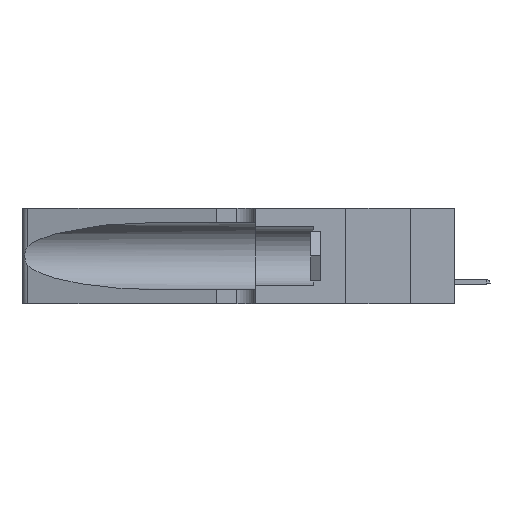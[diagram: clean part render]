
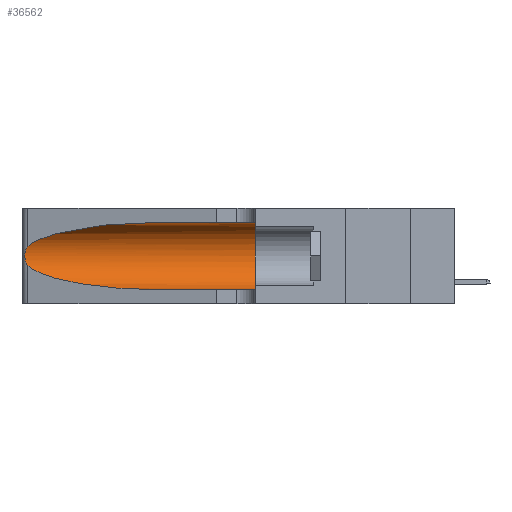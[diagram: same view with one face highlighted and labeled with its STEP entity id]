
A CAD part, left-side view. The second image highlights one B-rep face of the part: STEP entity #36562.
In plain terms, the highlighted cylindrical face has radius 3.308 mm (diameter 6.617 mm), a partial arc.
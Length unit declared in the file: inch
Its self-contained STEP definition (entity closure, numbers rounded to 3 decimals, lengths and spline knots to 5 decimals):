
#284 = VERTEX_POINT ( 'NONE', #16580 ) ;
#326 = EDGE_CURVE ( 'NONE', #35781, #31100, #12256, .T. ) ;
#497 = CARTESIAN_POINT ( 'NONE',  ( 0.25789, 1.23486, 0.15765 ) ) ;
#1213 = CARTESIAN_POINT ( 'NONE',  ( 0.25787, 1.23484, 0.2124 ) ) ;
#1489 = DIRECTION ( 'NONE',  ( 0., 0., 1. ) ) ;
#1950 = CARTESIAN_POINT ( 'NONE',  ( 0.1305, 0.35, 0.185 ) ) ;
#2249 = CARTESIAN_POINT ( 'NONE',  ( 0.25487, 1.22718, 0.14631 ) ) ;
#2952 = B_SPLINE_CURVE_WITH_KNOTS ( 'NONE', 3,
 ( #15940, #4539, #15233, #1213, #15704, #30435, #8803, #36635, #18561, #33062, #497, #14991, #29493, #22358 ),
 .UNSPECIFIED., .F., .F.,
 ( 4, 2, 2, 2, 2, 2, 4 ),
 ( 0., 0.00027, 0.00053, 0.00107, 0.0016, 0.00187, 0.00214 ),
 .UNSPECIFIED. ) ;
#3330 = CARTESIAN_POINT ( 'NONE',  ( 0.1305, 1.61858, 0.31525 ) ) ;
#4106 = EDGE_CURVE ( 'NONE', #16703, #284, #19844, .T. ) ;
#4110 = EDGE_CURVE ( 'NONE', #45057, #284, #41405, .T. ) ;
#4539 = CARTESIAN_POINT ( 'NONE',  ( 0.25555, 1.22994, 0.2215 ) ) ;
#5693 = CARTESIAN_POINT ( 'NONE',  ( 0.1305, 1.61858, 0.185 ) ) ;
#6502 = ORIENTED_EDGE ( 'NONE', *, *, #34901, .F. ) ;
#6588 = CARTESIAN_POINT ( 'NONE',  ( 0.1305, 0.35, 0.31525 ) ) ;
#7312 = EDGE_LOOP ( 'NONE', ( #26568, #13201, #28746, #25768, #24329, #6502 ) ) ;
#8803 = CARTESIAN_POINT ( 'NONE',  ( 0.26075, 1.23896, 0.19203 ) ) ;
#9600 = CARTESIAN_POINT ( 'NONE',  ( 0.2373, 1.15595, 0.08982 ) ) ;
#12256 =( BOUNDED_CURVE ( )  B_SPLINE_CURVE ( 3, ( #19680, #23252, #28396, #13670 ),
 .UNSPECIFIED., .F., .T. ) 
 B_SPLINE_CURVE_WITH_KNOTS ( ( 4, 4 ),
 ( 1.5708, 2.84003 ),
 .UNSPECIFIED. ) 
 CURVE ( )  GEOMETRIC_REPRESENTATION_ITEM ( )  RATIONAL_B_SPLINE_CURVE ( ( 1., 0.87, 0.87, 1. ) ) 
 REPRESENTATION_ITEM ( '' )  );
#13035 = CYLINDRICAL_SURFACE ( 'NONE', #34933, 0.13025 ) ;
#13201 = ORIENTED_EDGE ( 'NONE', *, *, #21586, .T. ) ;
#13670 = CARTESIAN_POINT ( 'NONE',  ( 0.25487, 1.22718, 0.22369 ) ) ;
#13685 = CARTESIAN_POINT ( 'NONE',  ( 0.1305, 0.72297, 0.05475 ) ) ;
#13928 = VERTEX_POINT ( 'NONE', #26891 ) ;
#14224 = CARTESIAN_POINT ( 'NONE',  ( 0.25487, 1.22718, 0.22369 ) ) ;
#14991 = CARTESIAN_POINT ( 'NONE',  ( 0.25639, 1.23186, 0.15144 ) ) ;
#15233 = CARTESIAN_POINT ( 'NONE',  ( 0.25639, 1.23184, 0.21858 ) ) ;
#15704 = CARTESIAN_POINT ( 'NONE',  ( 0.25854, 1.2359, 0.20912 ) ) ;
#15940 = CARTESIAN_POINT ( 'NONE',  ( 0.25487, 1.22718, 0.22369 ) ) ;
#16580 = CARTESIAN_POINT ( 'NONE',  ( 0.1305, 0.35, 0.05475 ) ) ;
#16703 = VERTEX_POINT ( 'NONE', #6588 ) ;
#16738 = CARTESIAN_POINT ( 'NONE',  ( 0.18966, 0.96281, 0.05475 ) ) ;
#18356 = CARTESIAN_POINT ( 'NONE',  ( 0.1305, 0.72297, 0.31525 ) ) ;
#18561 = CARTESIAN_POINT ( 'NONE',  ( 0.26017, 1.23833, 0.17102 ) ) ;
#19680 = CARTESIAN_POINT ( 'NONE',  ( 0.1305, 0.72297, 0.31525 ) ) ;
#19844 = CIRCLE ( 'NONE', #27442, 0.13025 ) ;
#20408 = DIRECTION ( 'NONE',  ( 0., -1., 0. ) ) ;
#20485 = CARTESIAN_POINT ( 'NONE',  ( 0.1305, 1.61858, 0.05475 ) ) ;
#20873 = FACE_OUTER_BOUND ( 'NONE', #7312, .T. ) ;
#21586 = EDGE_CURVE ( 'NONE', #31100, #13928, #2952, .T. ) ;
#22358 = CARTESIAN_POINT ( 'NONE',  ( 0.25487, 1.22718, 0.14631 ) ) ;
#23252 = CARTESIAN_POINT ( 'NONE',  ( 0.18966, 0.96281, 0.31525 ) ) ;
#24329 = ORIENTED_EDGE ( 'NONE', *, *, #4106, .F. ) ;
#25768 = ORIENTED_EDGE ( 'NONE', *, *, #4110, .T. ) ;
#25909 = VECTOR ( 'NONE', #27377, 39.37008 ) ;
#26554 =( BOUNDED_CURVE ( )  B_SPLINE_CURVE ( 3, ( #2249, #9600, #16738, #35038 ),
 .UNSPECIFIED., .F., .T. ) 
 B_SPLINE_CURVE_WITH_KNOTS ( ( 4, 4 ),
 ( 3.44316, 4.71239 ),
 .UNSPECIFIED. ) 
 CURVE ( )  GEOMETRIC_REPRESENTATION_ITEM ( )  RATIONAL_B_SPLINE_CURVE ( ( 1., 0.87, 0.87, 1. ) ) 
 REPRESENTATION_ITEM ( '' )  );
#26568 = ORIENTED_EDGE ( 'NONE', *, *, #326, .T. ) ;
#26891 = CARTESIAN_POINT ( 'NONE',  ( 0.25487, 1.22718, 0.14631 ) ) ;
#27377 = DIRECTION ( 'NONE',  ( 0., -1., 0. ) ) ;
#27442 = AXIS2_PLACEMENT_3D ( 'NONE', #1950, #34737, #1489 ) ;
#28396 = CARTESIAN_POINT ( 'NONE',  ( 0.2373, 1.15595, 0.28018 ) ) ;
#28740 = DIRECTION ( 'NONE',  ( 0., -1., 0. ) ) ;
#28746 = ORIENTED_EDGE ( 'NONE', *, *, #30209, .T. ) ;
#29493 = CARTESIAN_POINT ( 'NONE',  ( 0.25555, 1.22993, 0.14849 ) ) ;
#30209 = EDGE_CURVE ( 'NONE', #13928, #45057, #26554, .T. ) ;
#30435 = CARTESIAN_POINT ( 'NONE',  ( 0.26018, 1.23835, 0.19895 ) ) ;
#31100 = VERTEX_POINT ( 'NONE', #14224 ) ;
#33062 = CARTESIAN_POINT ( 'NONE',  ( 0.25856, 1.23593, 0.16098 ) ) ;
#34737 = DIRECTION ( 'NONE',  ( 0., 1., 0. ) ) ;
#34901 = EDGE_CURVE ( 'NONE', #35781, #16703, #38047, .T. ) ;
#34933 = AXIS2_PLACEMENT_3D ( 'NONE', #5693, #20408, #42267 ) ;
#35038 = CARTESIAN_POINT ( 'NONE',  ( 0.1305, 0.72297, 0.05475 ) ) ;
#35781 = VERTEX_POINT ( 'NONE', #18356 ) ;
#36469 = VECTOR ( 'NONE', #28740, 39.37008 ) ;
#36562 = ADVANCED_FACE ( 'NONE', ( #20873 ), #13035, .F. ) ;
#36635 = CARTESIAN_POINT ( 'NONE',  ( 0.26075, 1.23896, 0.178 ) ) ;
#38047 = LINE ( 'NONE', #3330, #36469 ) ;
#41405 = LINE ( 'NONE', #20485, #25909 ) ;
#42267 = DIRECTION ( 'NONE',  ( 0., 0., -1. ) ) ;
#45057 = VERTEX_POINT ( 'NONE', #13685 ) ;
